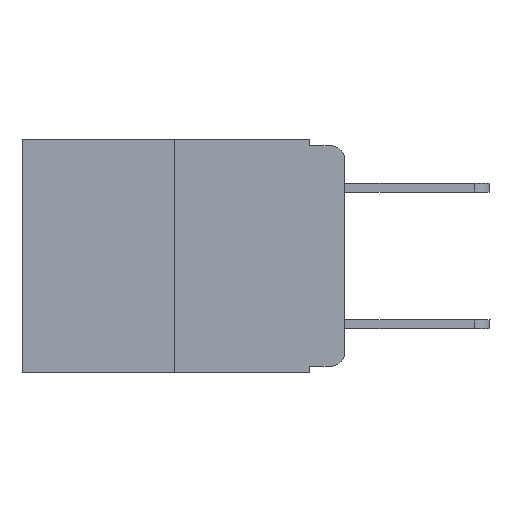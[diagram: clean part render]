
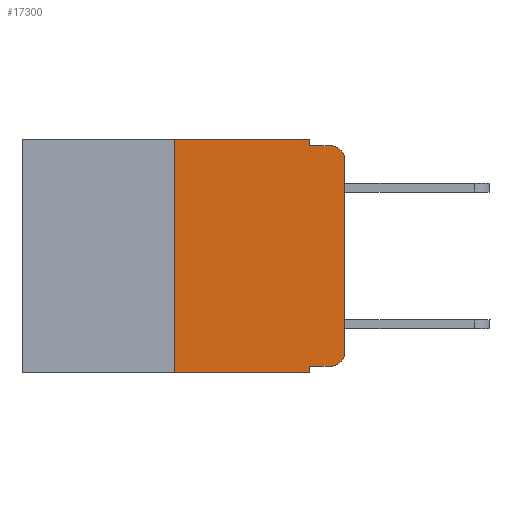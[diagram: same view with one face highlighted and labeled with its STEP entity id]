
A CAD part, left-side view. The second image highlights one B-rep face of the part: STEP entity #17300.
In plain terms, the highlighted planar face has unit normal (-1, 0, 0).
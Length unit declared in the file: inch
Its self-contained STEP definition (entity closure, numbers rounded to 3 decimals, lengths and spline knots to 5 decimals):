
#294 = VERTEX_POINT ( 'NONE', #13834 ) ;
#439 = VERTEX_POINT ( 'NONE', #6904 ) ;
#447 = CARTESIAN_POINT ( 'NONE',  ( 0., 0., 0. ) ) ;
#745 = CARTESIAN_POINT ( 'NONE',  ( 0., 0.25, -0.343 ) ) ;
#889 = ORIENTED_EDGE ( 'NONE', *, *, #8760, .F. ) ;
#1135 = ORIENTED_EDGE ( 'NONE', *, *, #23013, .F. ) ;
#1681 = DIRECTION ( 'NONE',  ( 1., 0., 0. ) ) ;
#1687 = EDGE_CURVE ( 'NONE', #12294, #5054, #3704, .T. ) ;
#1814 = ORIENTED_EDGE ( 'NONE', *, *, #12537, .T. ) ;
#2274 = DIRECTION ( 'NONE',  ( -1., 0., 0. ) ) ;
#2302 = EDGE_CURVE ( 'NONE', #439, #10469, #20447, .T. ) ;
#2422 = LINE ( 'NONE', #18785, #8708 ) ;
#2442 = ORIENTED_EDGE ( 'NONE', *, *, #21832, .T. ) ;
#2472 = DIRECTION ( 'NONE',  ( 0., -1., 0. ) ) ;
#3447 = CARTESIAN_POINT ( 'NONE',  ( 0., 0.25, 0. ) ) ;
#3704 = LINE ( 'NONE', #6559, #4887 ) ;
#4410 = VERTEX_POINT ( 'NONE', #22144 ) ;
#4414 = LINE ( 'NONE', #21448, #13975 ) ;
#4887 = VECTOR ( 'NONE', #6490, 39.37008 ) ;
#5054 = VERTEX_POINT ( 'NONE', #3447 ) ;
#5062 = EDGE_CURVE ( 'NONE', #10469, #21050, #5068, .T. ) ;
#5068 = CIRCLE ( 'NONE', #6830, 0.02 ) ;
#5617 = DIRECTION ( 'NONE',  ( 0., -1., 0. ) ) ;
#6490 = DIRECTION ( 'NONE',  ( 0., 0., 1. ) ) ;
#6559 = CARTESIAN_POINT ( 'NONE',  ( 0., 0.25, 0. ) ) ;
#6830 = AXIS2_PLACEMENT_3D ( 'NONE', #10877, #16824, #18746 ) ;
#6904 = CARTESIAN_POINT ( 'NONE',  ( 0., 0., -0.313 ) ) ;
#7183 = LINE ( 'NONE', #18777, #10790 ) ;
#7651 = VERTEX_POINT ( 'NONE', #16990 ) ;
#7871 = EDGE_CURVE ( 'NONE', #4410, #439, #11506, .T. ) ;
#7904 = DIRECTION ( 'NONE',  ( 0., -1., 0. ) ) ;
#8708 = VECTOR ( 'NONE', #5617, 39.37008 ) ;
#8760 = EDGE_CURVE ( 'NONE', #294, #21050, #15630, .T. ) ;
#8935 = CARTESIAN_POINT ( 'NONE',  ( 0., 0.02, -0.01 ) ) ;
#9261 = FACE_OUTER_BOUND ( 'NONE', #18289, .T. ) ;
#9962 = DIRECTION ( 'NONE',  ( 0., 0., -1. ) ) ;
#10217 = DIRECTION ( 'NONE',  ( 0., 0., 1. ) ) ;
#10469 = VERTEX_POINT ( 'NONE', #14009 ) ;
#10790 = VECTOR ( 'NONE', #24498, 39.37008 ) ;
#10865 = PLANE ( 'NONE',  #21355 ) ;
#10877 = CARTESIAN_POINT ( 'NONE',  ( 0., 0.02, -0.03 ) ) ;
#11309 = CARTESIAN_POINT ( 'NONE',  ( 0., 0.051, 0. ) ) ;
#11506 = CIRCLE ( 'NONE', #16333, 0.02 ) ;
#11521 = ORIENTED_EDGE ( 'NONE', *, *, #1687, .F. ) ;
#12294 = VERTEX_POINT ( 'NONE', #745 ) ;
#12537 = EDGE_CURVE ( 'NONE', #12294, #18526, #4414, .T. ) ;
#13115 = EDGE_CURVE ( 'NONE', #5054, #19549, #18756, .T. ) ;
#13834 = CARTESIAN_POINT ( 'NONE',  ( 0., 0.051, -0.01 ) ) ;
#13975 = VECTOR ( 'NONE', #14071, 39.37008 ) ;
#14009 = CARTESIAN_POINT ( 'NONE',  ( 0., 0., -0.03 ) ) ;
#14071 = DIRECTION ( 'NONE',  ( 0., -1., 0. ) ) ;
#14582 = ORIENTED_EDGE ( 'NONE', *, *, #2302, .T. ) ;
#15541 = ORIENTED_EDGE ( 'NONE', *, *, #7871, .T. ) ;
#15630 = LINE ( 'NONE', #15921, #24300 ) ;
#15921 = CARTESIAN_POINT ( 'NONE',  ( 0., 0.051, -0.01 ) ) ;
#16147 = CARTESIAN_POINT ( 'NONE',  ( 0., 0.051, 0. ) ) ;
#16333 = AXIS2_PLACEMENT_3D ( 'NONE', #21563, #2274, #9962 ) ;
#16617 = ORIENTED_EDGE ( 'NONE', *, *, #22976, .F. ) ;
#16824 = DIRECTION ( 'NONE',  ( -1., 0., 0. ) ) ;
#16835 = VECTOR ( 'NONE', #10217, 39.37008 ) ;
#16934 = DIRECTION ( 'NONE',  ( 0., 0., -1. ) ) ;
#16990 = CARTESIAN_POINT ( 'NONE',  ( 0., 0.051, -0.333 ) ) ;
#17300 = ADVANCED_FACE ( 'NONE', ( #9261 ), #10865, .F. ) ;
#17963 = VECTOR ( 'NONE', #16934, 39.37008 ) ;
#18289 = EDGE_LOOP ( 'NONE', ( #14582, #19547, #889, #16617, #19202, #11521, #1814, #1135, #2442, #15541 ) ) ;
#18526 = VERTEX_POINT ( 'NONE', #20444 ) ;
#18746 = DIRECTION ( 'NONE',  ( 0., 0., -1. ) ) ;
#18756 = LINE ( 'NONE', #21068, #21728 ) ;
#18777 = CARTESIAN_POINT ( 'NONE',  ( 0., 0.051, 0. ) ) ;
#18785 = CARTESIAN_POINT ( 'NONE',  ( 0., 0.051, -0.333 ) ) ;
#19202 = ORIENTED_EDGE ( 'NONE', *, *, #13115, .F. ) ;
#19547 = ORIENTED_EDGE ( 'NONE', *, *, #5062, .T. ) ;
#19549 = VERTEX_POINT ( 'NONE', #16147 ) ;
#20444 = CARTESIAN_POINT ( 'NONE',  ( 0., 0.051, -0.343 ) ) ;
#20447 = LINE ( 'NONE', #447, #16835 ) ;
#20750 = CARTESIAN_POINT ( 'NONE',  ( 0., 0.473, 0. ) ) ;
#21050 = VERTEX_POINT ( 'NONE', #8935 ) ;
#21068 = CARTESIAN_POINT ( 'NONE',  ( 0., 0.473, 0. ) ) ;
#21355 = AXIS2_PLACEMENT_3D ( 'NONE', #20750, #1681, #24213 ) ;
#21448 = CARTESIAN_POINT ( 'NONE',  ( 0., 0.473, -0.343 ) ) ;
#21563 = CARTESIAN_POINT ( 'NONE',  ( 0., 0.02, -0.313 ) ) ;
#21728 = VECTOR ( 'NONE', #7904, 39.37008 ) ;
#21832 = EDGE_CURVE ( 'NONE', #7651, #4410, #2422, .T. ) ;
#22144 = CARTESIAN_POINT ( 'NONE',  ( 0., 0.02, -0.333 ) ) ;
#22460 = LINE ( 'NONE', #11309, #17963 ) ;
#22976 = EDGE_CURVE ( 'NONE', #19549, #294, #22460, .T. ) ;
#23013 = EDGE_CURVE ( 'NONE', #7651, #18526, #7183, .T. ) ;
#24213 = DIRECTION ( 'NONE',  ( 0., 0., -1. ) ) ;
#24300 = VECTOR ( 'NONE', #2472, 39.37008 ) ;
#24498 = DIRECTION ( 'NONE',  ( 0., 0., -1. ) ) ;
